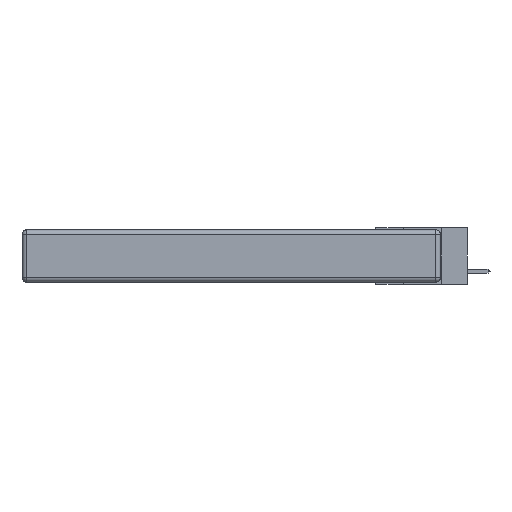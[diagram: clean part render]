
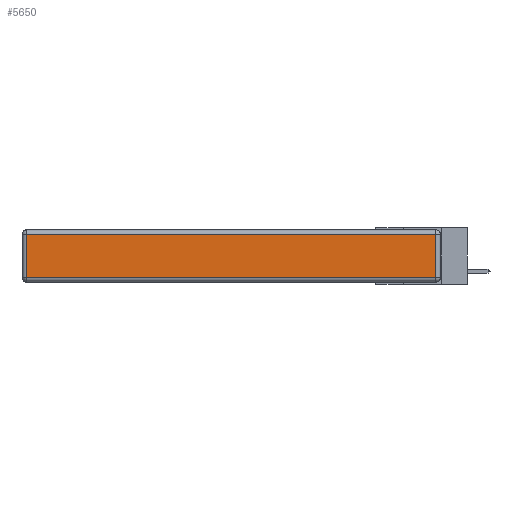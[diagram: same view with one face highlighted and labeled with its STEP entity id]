
A CAD part, left-side view. The second image highlights one B-rep face of the part: STEP entity #5650.
In plain terms, the highlighted planar face has unit normal (-1, 0, 0).
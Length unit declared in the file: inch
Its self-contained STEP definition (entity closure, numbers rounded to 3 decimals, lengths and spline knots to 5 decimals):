
#6 = PLANE ( 'NONE',  #9141 ) ;
#130 = CARTESIAN_POINT ( 'NONE',  ( 0., 0.03, -0.343 ) ) ;
#961 = CARTESIAN_POINT ( 'NONE',  ( 0., 0.03, -0.313 ) ) ;
#1119 = CARTESIAN_POINT ( 'NONE',  ( 0., 0., -0.313 ) ) ;
#1328 = CARTESIAN_POINT ( 'NONE',  ( 0., 2.75, -0.03 ) ) ;
#1517 = CARTESIAN_POINT ( 'NONE',  ( 0., 0., -0.343 ) ) ;
#2911 = EDGE_CURVE ( 'NONE', #14472, #8702, #18443, .T. ) ;
#3165 = VECTOR ( 'NONE', #10012, 39.37008 ) ;
#3287 = DIRECTION ( 'NONE',  ( 0., 0., -1. ) ) ;
#3654 = VECTOR ( 'NONE', #3287, 39.37008 ) ;
#4137 = LINE ( 'NONE', #15201, #3654 ) ;
#4263 = VERTEX_POINT ( 'NONE', #961 ) ;
#5164 = EDGE_CURVE ( 'NONE', #8702, #12500, #4137, .T. ) ;
#5650 = ADVANCED_FACE ( 'NONE', ( #6466 ), #6, .T. ) ;
#6466 = FACE_OUTER_BOUND ( 'NONE', #13667, .T. ) ;
#8474 = ORIENTED_EDGE ( 'NONE', *, *, #5164, .T. ) ;
#8702 = VERTEX_POINT ( 'NONE', #12120 ) ;
#9141 = AXIS2_PLACEMENT_3D ( 'NONE', #1517, #11990, #12065 ) ;
#9174 = DIRECTION ( 'NONE',  ( 0., 0., 1. ) ) ;
#10012 = DIRECTION ( 'NONE',  ( 0., -1., 0. ) ) ;
#11707 = ORIENTED_EDGE ( 'NONE', *, *, #18931, .T. ) ;
#11990 = DIRECTION ( 'NONE',  ( -1., 0., 0. ) ) ;
#12065 = DIRECTION ( 'NONE',  ( 0., 0., 1. ) ) ;
#12120 = CARTESIAN_POINT ( 'NONE',  ( 0., 2.72, -0.03 ) ) ;
#12500 = VERTEX_POINT ( 'NONE', #14252 ) ;
#13196 = DIRECTION ( 'NONE',  ( 0., 1., 0. ) ) ;
#13667 = EDGE_LOOP ( 'NONE', ( #11707, #14720, #15169, #8474 ) ) ;
#14252 = CARTESIAN_POINT ( 'NONE',  ( 0., 2.72, -0.313 ) ) ;
#14472 = VERTEX_POINT ( 'NONE', #16470 ) ;
#14720 = ORIENTED_EDGE ( 'NONE', *, *, #15945, .T. ) ;
#15169 = ORIENTED_EDGE ( 'NONE', *, *, #2911, .T. ) ;
#15201 = CARTESIAN_POINT ( 'NONE',  ( 0., 2.72, -0.343 ) ) ;
#15850 = VECTOR ( 'NONE', #13196, 39.37008 ) ;
#15945 = EDGE_CURVE ( 'NONE', #4263, #14472, #18974, .T. ) ;
#16285 = LINE ( 'NONE', #1119, #3165 ) ;
#16470 = CARTESIAN_POINT ( 'NONE',  ( 0., 0.03, -0.03 ) ) ;
#17550 = VECTOR ( 'NONE', #9174, 39.37008 ) ;
#18443 = LINE ( 'NONE', #1328, #15850 ) ;
#18931 = EDGE_CURVE ( 'NONE', #12500, #4263, #16285, .T. ) ;
#18974 = LINE ( 'NONE', #130, #17550 ) ;
